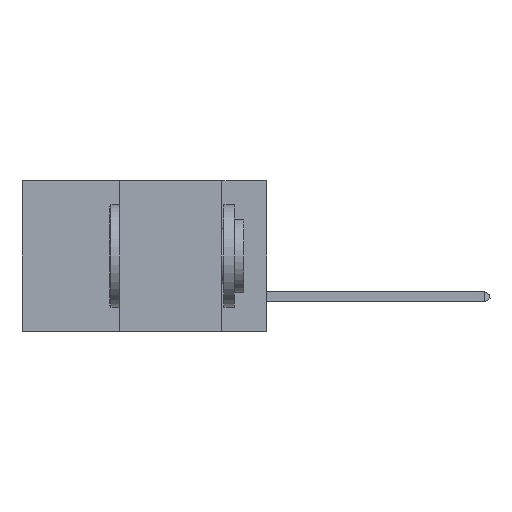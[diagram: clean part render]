
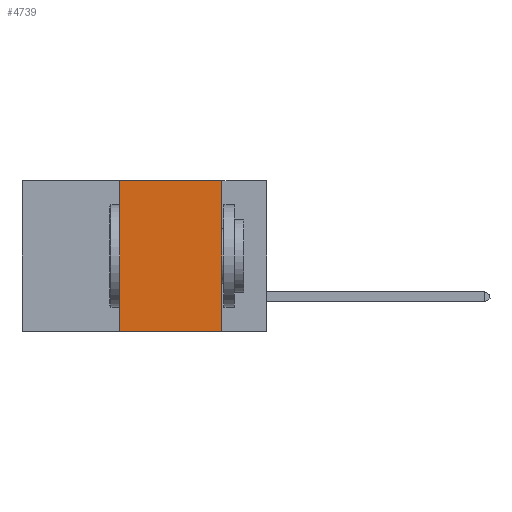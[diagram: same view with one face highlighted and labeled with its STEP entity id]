
A CAD part, left-side view. The second image highlights one B-rep face of the part: STEP entity #4739.
In plain terms, the highlighted planar face has unit normal (-1, 0, 0).
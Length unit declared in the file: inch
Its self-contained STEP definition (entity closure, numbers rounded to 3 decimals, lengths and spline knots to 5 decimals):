
#355 = VECTOR ( 'NONE', #15529, 39.37008 ) ;
#2213 = ORIENTED_EDGE ( 'NONE', *, *, #3316, .F. ) ;
#2731 = VERTEX_POINT ( 'NONE', #3734 ) ;
#3316 = EDGE_CURVE ( 'NONE', #2731, #11850, #8550, .T. ) ;
#3349 = FACE_OUTER_BOUND ( 'NONE', #17369, .T. ) ;
#3734 = CARTESIAN_POINT ( 'NONE',  ( 0., 0.36, -0.37 ) ) ;
#4418 = VECTOR ( 'NONE', #14992, 39.37008 ) ;
#4739 = ADVANCED_FACE ( 'NONE', ( #3349 ), #14623, .F. ) ;
#5020 = VERTEX_POINT ( 'NONE', #12165 ) ;
#5201 = VECTOR ( 'NONE', #10722, 39.37008 ) ;
#5612 = VERTEX_POINT ( 'NONE', #5941 ) ;
#5941 = CARTESIAN_POINT ( 'NONE',  ( 0., 0.11, 0. ) ) ;
#8141 = CARTESIAN_POINT ( 'NONE',  ( 0., 0.6, 0. ) ) ;
#8216 = LINE ( 'NONE', #16375, #4418 ) ;
#8550 = LINE ( 'NONE', #15200, #355 ) ;
#8697 = ORIENTED_EDGE ( 'NONE', *, *, #17763, .F. ) ;
#9295 = CARTESIAN_POINT ( 'NONE',  ( 0., 0.36, 0. ) ) ;
#9456 = LINE ( 'NONE', #8141, #16327 ) ;
#9801 = LINE ( 'NONE', #14754, #5201 ) ;
#10722 = DIRECTION ( 'NONE',  ( 0., -1., 0. ) ) ;
#11615 = ORIENTED_EDGE ( 'NONE', *, *, #14018, .T. ) ;
#11850 = VERTEX_POINT ( 'NONE', #9295 ) ;
#11945 = EDGE_CURVE ( 'NONE', #5612, #5020, #8216, .T. ) ;
#12165 = CARTESIAN_POINT ( 'NONE',  ( 0., 0.11, -0.37 ) ) ;
#13098 = AXIS2_PLACEMENT_3D ( 'NONE', #14609, #14571, #14558 ) ;
#14018 = EDGE_CURVE ( 'NONE', #2731, #5020, #9801, .T. ) ;
#14558 = DIRECTION ( 'NONE',  ( 0., 0., -1. ) ) ;
#14571 = DIRECTION ( 'NONE',  ( 1., 0., 0. ) ) ;
#14609 = CARTESIAN_POINT ( 'NONE',  ( 0., 0.6, 0. ) ) ;
#14623 = PLANE ( 'NONE',  #13098 ) ;
#14754 = CARTESIAN_POINT ( 'NONE',  ( 0., 0.6, -0.37 ) ) ;
#14992 = DIRECTION ( 'NONE',  ( 0., 0., -1. ) ) ;
#15200 = CARTESIAN_POINT ( 'NONE',  ( 0., 0.36, 0. ) ) ;
#15529 = DIRECTION ( 'NONE',  ( 0., 0., 1. ) ) ;
#16327 = VECTOR ( 'NONE', #16345, 39.37008 ) ;
#16345 = DIRECTION ( 'NONE',  ( 0., -1., 0. ) ) ;
#16375 = CARTESIAN_POINT ( 'NONE',  ( 0., 0.11, 0. ) ) ;
#16822 = ORIENTED_EDGE ( 'NONE', *, *, #11945, .F. ) ;
#17369 = EDGE_LOOP ( 'NONE', ( #16822, #8697, #2213, #11615 ) ) ;
#17763 = EDGE_CURVE ( 'NONE', #11850, #5612, #9456, .T. ) ;
